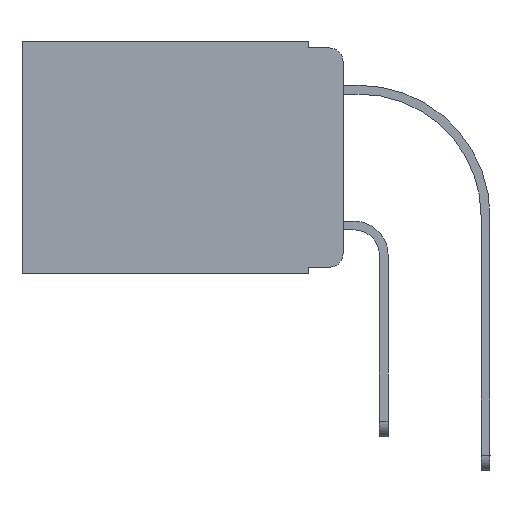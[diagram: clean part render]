
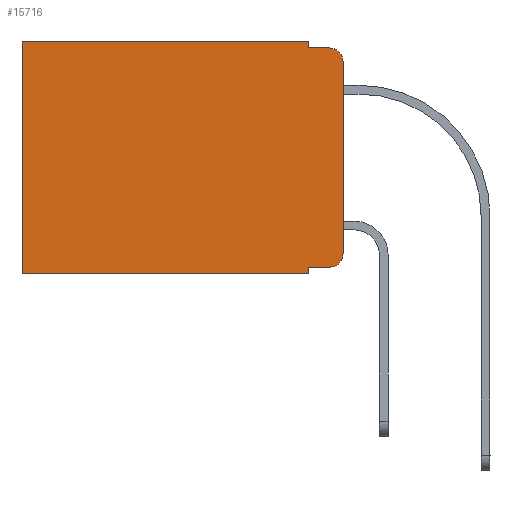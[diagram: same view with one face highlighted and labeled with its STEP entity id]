
A CAD part, left-side view. The second image highlights one B-rep face of the part: STEP entity #15716.
In plain terms, the highlighted planar face has unit normal (-1, 0, 0).
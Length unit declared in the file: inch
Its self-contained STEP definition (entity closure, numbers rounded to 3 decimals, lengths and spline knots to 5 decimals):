
#145 = AXIS2_PLACEMENT_3D ( 'NONE', #4468, #21772, #850 ) ;
#146 = LINE ( 'NONE', #21070, #20342 ) ;
#300 = DIRECTION ( 'NONE',  ( 0., 1., 0. ) ) ;
#355 = EDGE_CURVE ( 'NONE', #933, #8946, #2742, .T. ) ;
#472 = CARTESIAN_POINT ( 'NONE',  ( 0.298, 0.051, 0. ) ) ;
#515 = CARTESIAN_POINT ( 'NONE',  ( 0.298, 0., -0.313 ) ) ;
#596 = ORIENTED_EDGE ( 'NONE', *, *, #355, .T. ) ;
#720 = VECTOR ( 'NONE', #1059, 39.37008 ) ;
#785 = EDGE_CURVE ( 'NONE', #5291, #8955, #13044, .T. ) ;
#850 = DIRECTION ( 'NONE',  ( 0., 0., -1. ) ) ;
#933 = VERTEX_POINT ( 'NONE', #10745 ) ;
#940 = DIRECTION ( 'NONE',  ( 0., 0., -1. ) ) ;
#1023 = CARTESIAN_POINT ( 'NONE',  ( 0.298, 0.051, -0.01 ) ) ;
#1059 = DIRECTION ( 'NONE',  ( 0., 0., -1. ) ) ;
#2157 = AXIS2_PLACEMENT_3D ( 'NONE', #2567, #9495, #16411 ) ;
#2431 = AXIS2_PLACEMENT_3D ( 'NONE', #10149, #4565, #5129 ) ;
#2567 = CARTESIAN_POINT ( 'NONE',  ( 0.298, 0.02, -0.313 ) ) ;
#2626 = ORIENTED_EDGE ( 'NONE', *, *, #785, .F. ) ;
#2708 = CARTESIAN_POINT ( 'NONE',  ( 0.298, 0.051, -0.01 ) ) ;
#2742 = LINE ( 'NONE', #6164, #14316 ) ;
#3471 = VECTOR ( 'NONE', #4187, 39.37008 ) ;
#3870 = CARTESIAN_POINT ( 'NONE',  ( 0.298, 0., -0.03 ) ) ;
#4176 = VECTOR ( 'NONE', #17823, 39.37008 ) ;
#4187 = DIRECTION ( 'NONE',  ( 0., -1., 0. ) ) ;
#4217 = VERTEX_POINT ( 'NONE', #515 ) ;
#4468 = CARTESIAN_POINT ( 'NONE',  ( 0.298, 0., 0. ) ) ;
#4565 = DIRECTION ( 'NONE',  ( -1., 0., 0. ) ) ;
#4679 = CIRCLE ( 'NONE', #2157, 0.02 ) ;
#5126 = CARTESIAN_POINT ( 'NONE',  ( 0.298, 0.051, -0.333 ) ) ;
#5129 = DIRECTION ( 'NONE',  ( 0., 0., -1. ) ) ;
#5151 = EDGE_CURVE ( 'NONE', #18487, #5291, #9097, .T. ) ;
#5234 = CARTESIAN_POINT ( 'NONE',  ( 0.298, 0.473, -0.343 ) ) ;
#5291 = VERTEX_POINT ( 'NONE', #1023 ) ;
#5853 = PLANE ( 'NONE',  #145 ) ;
#6164 = CARTESIAN_POINT ( 'NONE',  ( 0.298, 0.473, 0. ) ) ;
#6299 = VECTOR ( 'NONE', #300, 39.37008 ) ;
#7061 = LINE ( 'NONE', #5126, #8737 ) ;
#7378 = CARTESIAN_POINT ( 'NONE',  ( 0.298, 0.051, 0. ) ) ;
#7907 = FACE_OUTER_BOUND ( 'NONE', #11999, .T. ) ;
#8162 = VERTEX_POINT ( 'NONE', #12022 ) ;
#8727 = ORIENTED_EDGE ( 'NONE', *, *, #14086, .F. ) ;
#8737 = VECTOR ( 'NONE', #12048, 39.37008 ) ;
#8794 = ORIENTED_EDGE ( 'NONE', *, *, #20902, .F. ) ;
#8825 = EDGE_CURVE ( 'NONE', #10424, #8955, #18383, .T. ) ;
#8946 = VERTEX_POINT ( 'NONE', #5234 ) ;
#8955 = VERTEX_POINT ( 'NONE', #14430 ) ;
#9097 = LINE ( 'NONE', #7378, #4176 ) ;
#9495 = DIRECTION ( 'NONE',  ( -1., 0., 0. ) ) ;
#10149 = CARTESIAN_POINT ( 'NONE',  ( 0.298, 0.02, -0.03 ) ) ;
#10154 = ORIENTED_EDGE ( 'NONE', *, *, #14556, .T. ) ;
#10424 = VERTEX_POINT ( 'NONE', #3870 ) ;
#10745 = CARTESIAN_POINT ( 'NONE',  ( 0.298, 0.473, 0. ) ) ;
#10831 = CARTESIAN_POINT ( 'NONE',  ( 0.298, 0., -0.343 ) ) ;
#11460 = VERTEX_POINT ( 'NONE', #11875 ) ;
#11875 = CARTESIAN_POINT ( 'NONE',  ( 0.298, 0.051, -0.333 ) ) ;
#11999 = EDGE_LOOP ( 'NONE', ( #22414, #17267, #2626, #20706, #16626, #596, #8794, #8727, #10154, #19256 ) ) ;
#12022 = CARTESIAN_POINT ( 'NONE',  ( 0.298, 0.02, -0.333 ) ) ;
#12048 = DIRECTION ( 'NONE',  ( 0., -1., 0. ) ) ;
#12604 = EDGE_CURVE ( 'NONE', #8162, #4217, #4679, .T. ) ;
#13044 = LINE ( 'NONE', #2708, #3471 ) ;
#13103 = EDGE_CURVE ( 'NONE', #10424, #4217, #16612, .T. ) ;
#14086 = EDGE_CURVE ( 'NONE', #11460, #20654, #146, .T. ) ;
#14118 = DIRECTION ( 'NONE',  ( 0., 0., -1. ) ) ;
#14316 = VECTOR ( 'NONE', #940, 39.37008 ) ;
#14386 = CARTESIAN_POINT ( 'NONE',  ( 0.298, 0.051, -0.343 ) ) ;
#14430 = CARTESIAN_POINT ( 'NONE',  ( 0.298, 0.02, -0.01 ) ) ;
#14556 = EDGE_CURVE ( 'NONE', #11460, #8162, #7061, .T. ) ;
#15311 = VECTOR ( 'NONE', #18818, 39.37008 ) ;
#15531 = EDGE_CURVE ( 'NONE', #18487, #933, #17439, .T. ) ;
#15716 = ADVANCED_FACE ( 'NONE', ( #7907 ), #5853, .F. ) ;
#16411 = DIRECTION ( 'NONE',  ( 0., 0., -1. ) ) ;
#16612 = LINE ( 'NONE', #22078, #720 ) ;
#16626 = ORIENTED_EDGE ( 'NONE', *, *, #15531, .T. ) ;
#17267 = ORIENTED_EDGE ( 'NONE', *, *, #8825, .T. ) ;
#17439 = LINE ( 'NONE', #17673, #6299 ) ;
#17673 = CARTESIAN_POINT ( 'NONE',  ( 0.298, 0., 0. ) ) ;
#17823 = DIRECTION ( 'NONE',  ( 0., 0., -1. ) ) ;
#18383 = CIRCLE ( 'NONE', #2431, 0.02 ) ;
#18487 = VERTEX_POINT ( 'NONE', #472 ) ;
#18818 = DIRECTION ( 'NONE',  ( 0., 1., 0. ) ) ;
#19256 = ORIENTED_EDGE ( 'NONE', *, *, #12604, .T. ) ;
#20342 = VECTOR ( 'NONE', #14118, 39.37008 ) ;
#20654 = VERTEX_POINT ( 'NONE', #14386 ) ;
#20706 = ORIENTED_EDGE ( 'NONE', *, *, #5151, .F. ) ;
#20902 = EDGE_CURVE ( 'NONE', #20654, #8946, #22344, .T. ) ;
#21070 = CARTESIAN_POINT ( 'NONE',  ( 0.298, 0.051, 0. ) ) ;
#21772 = DIRECTION ( 'NONE',  ( 1., 0., 0. ) ) ;
#22078 = CARTESIAN_POINT ( 'NONE',  ( 0.298, 0., 0. ) ) ;
#22344 = LINE ( 'NONE', #10831, #15311 ) ;
#22414 = ORIENTED_EDGE ( 'NONE', *, *, #13103, .F. ) ;
